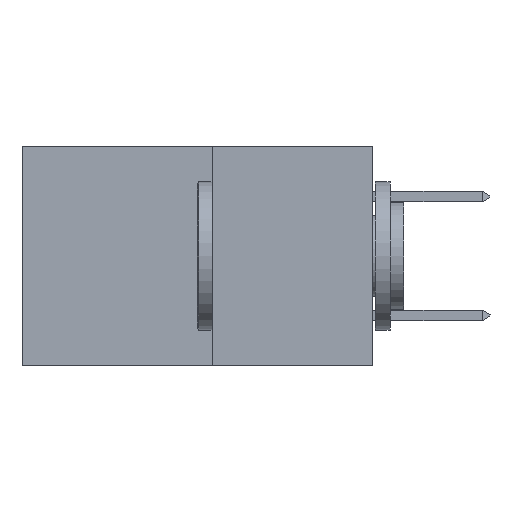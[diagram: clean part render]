
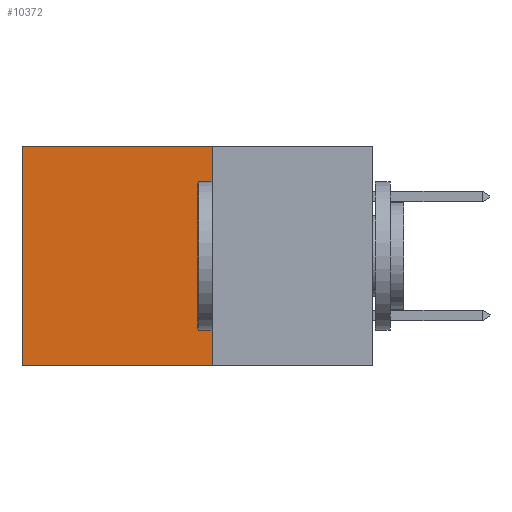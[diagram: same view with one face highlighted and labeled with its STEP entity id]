
A CAD part, left-side view. The second image highlights one B-rep face of the part: STEP entity #10372.
In plain terms, the highlighted planar face has unit normal (-1, 0, 0).
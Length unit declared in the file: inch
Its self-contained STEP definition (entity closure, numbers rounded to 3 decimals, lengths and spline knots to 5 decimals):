
#95 = VECTOR ( 'NONE', #10675, 39.37008 ) ;
#1648 = EDGE_CURVE ( 'NONE', #20304, #20592, #10793, .T. ) ;
#2207 = DIRECTION ( 'NONE',  ( 0., 1., 0. ) ) ;
#3140 = CARTESIAN_POINT ( 'NONE',  ( 0.277, 0.59, -0.37 ) ) ;
#4146 = VECTOR ( 'NONE', #5642, 39.37008 ) ;
#4675 = LINE ( 'NONE', #3140, #95 ) ;
#5619 = CARTESIAN_POINT ( 'NONE',  ( 0.277, 0.27, -0.37 ) ) ;
#5642 = DIRECTION ( 'NONE',  ( 0., 0., -1. ) ) ;
#5770 = VECTOR ( 'NONE', #11819, 39.37008 ) ;
#5789 = CARTESIAN_POINT ( 'NONE',  ( 0.277, 0.27, -0.37 ) ) ;
#6061 = ORIENTED_EDGE ( 'NONE', *, *, #22620, .F. ) ;
#6436 = ORIENTED_EDGE ( 'NONE', *, *, #19044, .F. ) ;
#7572 = CARTESIAN_POINT ( 'NONE',  ( 0.277, 0.27, 0. ) ) ;
#7693 = DIRECTION ( 'NONE',  ( 0., 0., -1. ) ) ;
#7831 = ORIENTED_EDGE ( 'NONE', *, *, #1648, .T. ) ;
#10372 = ADVANCED_FACE ( 'NONE', ( #11620 ), #17095, .F. ) ;
#10675 = DIRECTION ( 'NONE',  ( 0., 0., -1. ) ) ;
#10793 = LINE ( 'NONE', #7572, #5770 ) ;
#11620 = FACE_OUTER_BOUND ( 'NONE', #17748, .T. ) ;
#11654 = CARTESIAN_POINT ( 'NONE',  ( 0.277, 0.27, -0.37 ) ) ;
#11819 = DIRECTION ( 'NONE',  ( 0., 1., 0. ) ) ;
#13545 = CARTESIAN_POINT ( 'NONE',  ( 0.277, 0.59, -0.37 ) ) ;
#13708 = AXIS2_PLACEMENT_3D ( 'NONE', #5789, #18995, #7693 ) ;
#14166 = EDGE_CURVE ( 'NONE', #20592, #22623, #4675, .T. ) ;
#14271 = VERTEX_POINT ( 'NONE', #5619 ) ;
#16953 = CARTESIAN_POINT ( 'NONE',  ( 0.277, 0.27, -0.37 ) ) ;
#17095 = PLANE ( 'NONE',  #13708 ) ;
#17746 = ORIENTED_EDGE ( 'NONE', *, *, #14166, .T. ) ;
#17748 = EDGE_LOOP ( 'NONE', ( #17746, #6061, #6436, #7831 ) ) ;
#18084 = LINE ( 'NONE', #16953, #4146 ) ;
#18995 = DIRECTION ( 'NONE',  ( 1., 0., 0. ) ) ;
#19044 = EDGE_CURVE ( 'NONE', #20304, #14271, #18084, .T. ) ;
#19146 = LINE ( 'NONE', #11654, #23603 ) ;
#20304 = VERTEX_POINT ( 'NONE', #23778 ) ;
#20592 = VERTEX_POINT ( 'NONE', #22660 ) ;
#22620 = EDGE_CURVE ( 'NONE', #14271, #22623, #19146, .T. ) ;
#22623 = VERTEX_POINT ( 'NONE', #13545 ) ;
#22660 = CARTESIAN_POINT ( 'NONE',  ( 0.277, 0.59, 0. ) ) ;
#23603 = VECTOR ( 'NONE', #2207, 39.37008 ) ;
#23778 = CARTESIAN_POINT ( 'NONE',  ( 0.277, 0.27, 0. ) ) ;
